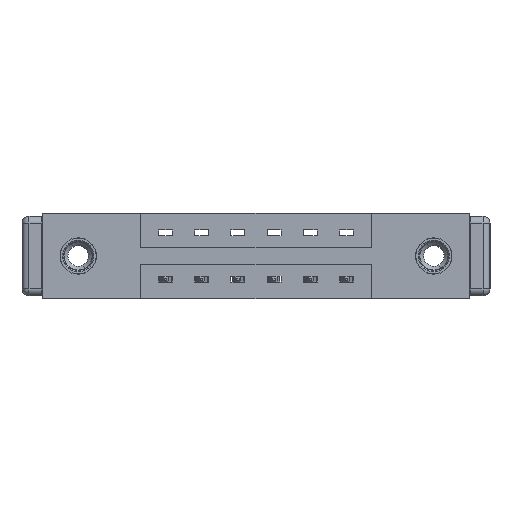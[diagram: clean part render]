
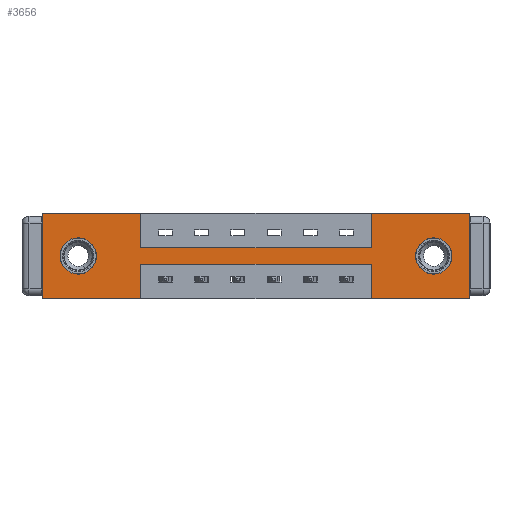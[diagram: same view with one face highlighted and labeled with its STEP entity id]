
A CAD part, front view. The second image highlights one B-rep face of the part: STEP entity #3656.
In plain terms, the highlighted planar face has unit normal (0, -1, 0).
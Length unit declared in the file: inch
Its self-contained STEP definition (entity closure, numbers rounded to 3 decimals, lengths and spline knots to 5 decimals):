
#95 = EDGE_CURVE ( 'NONE', #5404, #823, #560, .T. ) ;
#125 = VERTEX_POINT ( 'NONE', #7134 ) ;
#153 = ORIENTED_EDGE ( 'NONE', *, *, #8197, .F. ) ;
#188 = LINE ( 'NONE', #6750, #7507 ) ;
#326 = CIRCLE ( 'NONE', #6230, 0.078 ) ;
#330 = ORIENTED_EDGE ( 'NONE', *, *, #1349, .F. ) ;
#359 = ORIENTED_EDGE ( 'NONE', *, *, #10274, .F. ) ;
#480 = EDGE_CURVE ( 'NONE', #9215, #3305, #4410, .T. ) ;
#504 = CARTESIAN_POINT ( 'NONE',  ( 0., 0., 0. ) ) ;
#519 = CARTESIAN_POINT ( 'NONE',  ( 1.417, 0., -0.15 ) ) ;
#555 = VECTOR ( 'NONE', #3935, 39.37008 ) ;
#560 = LINE ( 'NONE', #1559, #9749 ) ;
#619 = ORIENTED_EDGE ( 'NONE', *, *, #2495, .F. ) ;
#646 = CARTESIAN_POINT ( 'NONE',  ( 0., 0., 0. ) ) ;
#762 = EDGE_CURVE ( 'NONE', #7553, #10965, #1373, .T. ) ;
#823 = VERTEX_POINT ( 'NONE', #11478 ) ;
#871 = CARTESIAN_POINT ( 'NONE',  ( 0.155, 0., -0.185 ) ) ;
#921 = DIRECTION ( 'NONE',  ( 0., 0., -1. ) ) ;
#1019 = FACE_OUTER_BOUND ( 'NONE', #3619, .T. ) ;
#1062 = LINE ( 'NONE', #2661, #10570 ) ;
#1277 = DIRECTION ( 'NONE',  ( 0., -1., 0. ) ) ;
#1349 = EDGE_CURVE ( 'NONE', #6822, #11516, #9712, .T. ) ;
#1373 = CIRCLE ( 'NONE', #1609, 0.078 ) ;
#1479 = LINE ( 'NONE', #6833, #2194 ) ;
#1559 = CARTESIAN_POINT ( 'NONE',  ( 0.425, 0., 0. ) ) ;
#1609 = AXIS2_PLACEMENT_3D ( 'NONE', #8717, #2347, #4288 ) ;
#1665 = CARTESIAN_POINT ( 'NONE',  ( 1.417, 0., -0.22 ) ) ;
#1666 = ORIENTED_EDGE ( 'NONE', *, *, #7916, .F. ) ;
#1713 = DIRECTION ( 'NONE',  ( 0., 0., -1. ) ) ;
#1727 = VERTEX_POINT ( 'NONE', #7139 ) ;
#1804 = EDGE_CURVE ( 'NONE', #8962, #1727, #6522, .T. ) ;
#1873 = LINE ( 'NONE', #9604, #8502 ) ;
#2034 = CARTESIAN_POINT ( 'NONE',  ( 1.417, 0., 0. ) ) ;
#2094 = DIRECTION ( 'NONE',  ( 0., 0., 1. ) ) ;
#2099 = DIRECTION ( 'NONE',  ( -1., 0., 0. ) ) ;
#2194 = VECTOR ( 'NONE', #2256, 39.37008 ) ;
#2211 = VECTOR ( 'NONE', #6171, 39.37008 ) ;
#2256 = DIRECTION ( 'NONE',  ( 0., 0., -1. ) ) ;
#2257 = VERTEX_POINT ( 'NONE', #3388 ) ;
#2347 = DIRECTION ( 'NONE',  ( 0., 1., 0. ) ) ;
#2495 = EDGE_CURVE ( 'NONE', #125, #8962, #1479, .T. ) ;
#2633 = VECTOR ( 'NONE', #11710, 39.37008 ) ;
#2648 = CARTESIAN_POINT ( 'NONE',  ( 0., 0., 0. ) ) ;
#2661 = CARTESIAN_POINT ( 'NONE',  ( 1.842, 0., 0. ) ) ;
#2691 = CARTESIAN_POINT ( 'NONE',  ( 1.417, 0., -0.37 ) ) ;
#2717 = DIRECTION ( 'NONE',  ( 0., 0., 1. ) ) ;
#2992 = AXIS2_PLACEMENT_3D ( 'NONE', #8260, #11036, #9140 ) ;
#3060 = VERTEX_POINT ( 'NONE', #6633 ) ;
#3115 = DIRECTION ( 'NONE',  ( 0., 0., -1. ) ) ;
#3141 = DIRECTION ( 'NONE',  ( 1., 0., 0. ) ) ;
#3299 = LINE ( 'NONE', #7486, #3884 ) ;
#3305 = VERTEX_POINT ( 'NONE', #9691 ) ;
#3388 = CARTESIAN_POINT ( 'NONE',  ( 1.842, 0., 0. ) ) ;
#3540 = CARTESIAN_POINT ( 'NONE',  ( 0.425, 0., 0. ) ) ;
#3591 = DIRECTION ( 'NONE',  ( 1., 0., 0. ) ) ;
#3619 = EDGE_LOOP ( 'NONE', ( #619, #7927, #330, #9141, #153, #7302, #6827, #9240, #6252, #359, #1666, #6781 ) ) ;
#3656 = ADVANCED_FACE ( 'NONE', ( #10810, #5599, #1019 ), #7871, .T. ) ;
#3803 = EDGE_CURVE ( 'NONE', #11516, #125, #1873, .T. ) ;
#3884 = VECTOR ( 'NONE', #3141, 39.37008 ) ;
#3915 = CARTESIAN_POINT ( 'NONE',  ( 0.155, 0., -0.185 ) ) ;
#3935 = DIRECTION ( 'NONE',  ( 0., 0., 1. ) ) ;
#3959 = ORIENTED_EDGE ( 'NONE', *, *, #480, .T. ) ;
#4133 = DIRECTION ( 'NONE',  ( -1., 0., 0. ) ) ;
#4288 = DIRECTION ( 'NONE',  ( 0., 0., -1. ) ) ;
#4376 = CARTESIAN_POINT ( 'NONE',  ( 0., 0., -0.37 ) ) ;
#4410 = CIRCLE ( 'NONE', #11027, 0.078 ) ;
#4535 = CARTESIAN_POINT ( 'NONE',  ( 1.687, 0., -0.263 ) ) ;
#4813 = AXIS2_PLACEMENT_3D ( 'NONE', #8682, #1277, #3115 ) ;
#4834 = LINE ( 'NONE', #2034, #555 ) ;
#4891 = VECTOR ( 'NONE', #3591, 39.37008 ) ;
#4892 = DIRECTION ( 'NONE',  ( 0., 1., 0. ) ) ;
#5063 = EDGE_CURVE ( 'NONE', #823, #8583, #3299, .T. ) ;
#5197 = CIRCLE ( 'NONE', #2992, 0.078 ) ;
#5404 = VERTEX_POINT ( 'NONE', #3540 ) ;
#5487 = CARTESIAN_POINT ( 'NONE',  ( 1.687, 0., -0.107 ) ) ;
#5548 = ORIENTED_EDGE ( 'NONE', *, *, #8757, .T. ) ;
#5599 = FACE_BOUND ( 'NONE', #11301, .T. ) ;
#6006 = LINE ( 'NONE', #10924, #6585 ) ;
#6171 = DIRECTION ( 'NONE',  ( 0., 0., 1. ) ) ;
#6230 = AXIS2_PLACEMENT_3D ( 'NONE', #3915, #4892, #2094 ) ;
#6252 = ORIENTED_EDGE ( 'NONE', *, *, #95, .F. ) ;
#6364 = EDGE_CURVE ( 'NONE', #8583, #11296, #4834, .T. ) ;
#6522 = LINE ( 'NONE', #4376, #2633 ) ;
#6585 = VECTOR ( 'NONE', #11853, 39.37008 ) ;
#6594 = CARTESIAN_POINT ( 'NONE',  ( 0.425, 0., -0.37 ) ) ;
#6633 = CARTESIAN_POINT ( 'NONE',  ( 1.842, 0., -0.37 ) ) ;
#6750 = CARTESIAN_POINT ( 'NONE',  ( 0., 0., -0.37 ) ) ;
#6781 = ORIENTED_EDGE ( 'NONE', *, *, #1804, .F. ) ;
#6822 = VERTEX_POINT ( 'NONE', #2691 ) ;
#6827 = ORIENTED_EDGE ( 'NONE', *, *, #6364, .F. ) ;
#6833 = CARTESIAN_POINT ( 'NONE',  ( 0.425, 0., -0.37 ) ) ;
#7134 = CARTESIAN_POINT ( 'NONE',  ( 0.425, 0., -0.22 ) ) ;
#7139 = CARTESIAN_POINT ( 'NONE',  ( 0., 0., -0.37 ) ) ;
#7228 = CARTESIAN_POINT ( 'NONE',  ( 1.417, 0., -0.37 ) ) ;
#7288 = DIRECTION ( 'NONE',  ( 0., 0., 1. ) ) ;
#7302 = ORIENTED_EDGE ( 'NONE', *, *, #11585, .F. ) ;
#7393 = VERTEX_POINT ( 'NONE', #504 ) ;
#7486 = CARTESIAN_POINT ( 'NONE',  ( 0.425, 0., -0.15 ) ) ;
#7507 = VECTOR ( 'NONE', #2099, 39.37008 ) ;
#7553 = VERTEX_POINT ( 'NONE', #4535 ) ;
#7871 = PLANE ( 'NONE',  #4813 ) ;
#7916 = EDGE_CURVE ( 'NONE', #1727, #7393, #9844, .T. ) ;
#7927 = ORIENTED_EDGE ( 'NONE', *, *, #3803, .F. ) ;
#8030 = ORIENTED_EDGE ( 'NONE', *, *, #762, .T. ) ;
#8197 = EDGE_CURVE ( 'NONE', #2257, #3060, #1062, .T. ) ;
#8260 = CARTESIAN_POINT ( 'NONE',  ( 1.687, 0., -0.185 ) ) ;
#8271 = VECTOR ( 'NONE', #2717, 39.37008 ) ;
#8502 = VECTOR ( 'NONE', #4133, 39.37008 ) ;
#8583 = VERTEX_POINT ( 'NONE', #519 ) ;
#8682 = CARTESIAN_POINT ( 'NONE',  ( 0., 0., -0.37 ) ) ;
#8717 = CARTESIAN_POINT ( 'NONE',  ( 1.687, 0., -0.185 ) ) ;
#8757 = EDGE_CURVE ( 'NONE', #10965, #7553, #5197, .T. ) ;
#8901 = EDGE_CURVE ( 'NONE', #3060, #6822, #188, .T. ) ;
#8962 = VERTEX_POINT ( 'NONE', #6594 ) ;
#9140 = DIRECTION ( 'NONE',  ( 0., 0., -1. ) ) ;
#9141 = ORIENTED_EDGE ( 'NONE', *, *, #8901, .F. ) ;
#9215 = VERTEX_POINT ( 'NONE', #11581 ) ;
#9240 = ORIENTED_EDGE ( 'NONE', *, *, #5063, .F. ) ;
#9604 = CARTESIAN_POINT ( 'NONE',  ( 0.425, 0., -0.22 ) ) ;
#9650 = CARTESIAN_POINT ( 'NONE',  ( 1.417, 0., 0. ) ) ;
#9691 = CARTESIAN_POINT ( 'NONE',  ( 0.155, 0., -0.107 ) ) ;
#9712 = LINE ( 'NONE', #7228, #8271 ) ;
#9724 = ORIENTED_EDGE ( 'NONE', *, *, #10080, .T. ) ;
#9749 = VECTOR ( 'NONE', #1713, 39.37008 ) ;
#9844 = LINE ( 'NONE', #646, #2211 ) ;
#9949 = LINE ( 'NONE', #2648, #4891 ) ;
#10080 = EDGE_CURVE ( 'NONE', #3305, #9215, #326, .T. ) ;
#10274 = EDGE_CURVE ( 'NONE', #7393, #5404, #9949, .T. ) ;
#10570 = VECTOR ( 'NONE', #921, 39.37008 ) ;
#10807 = DIRECTION ( 'NONE',  ( 0., 1., 0. ) ) ;
#10810 = FACE_BOUND ( 'NONE', #11782, .T. ) ;
#10924 = CARTESIAN_POINT ( 'NONE',  ( 0., 0., 0. ) ) ;
#10965 = VERTEX_POINT ( 'NONE', #5487 ) ;
#11027 = AXIS2_PLACEMENT_3D ( 'NONE', #871, #10807, #7288 ) ;
#11036 = DIRECTION ( 'NONE',  ( 0., 1., 0. ) ) ;
#11296 = VERTEX_POINT ( 'NONE', #9650 ) ;
#11301 = EDGE_LOOP ( 'NONE', ( #9724, #3959 ) ) ;
#11478 = CARTESIAN_POINT ( 'NONE',  ( 0.425, 0., -0.15 ) ) ;
#11516 = VERTEX_POINT ( 'NONE', #1665 ) ;
#11581 = CARTESIAN_POINT ( 'NONE',  ( 0.155, 0., -0.263 ) ) ;
#11585 = EDGE_CURVE ( 'NONE', #11296, #2257, #6006, .T. ) ;
#11710 = DIRECTION ( 'NONE',  ( -1., 0., 0. ) ) ;
#11782 = EDGE_LOOP ( 'NONE', ( #5548, #8030 ) ) ;
#11853 = DIRECTION ( 'NONE',  ( 1., 0., 0. ) ) ;
